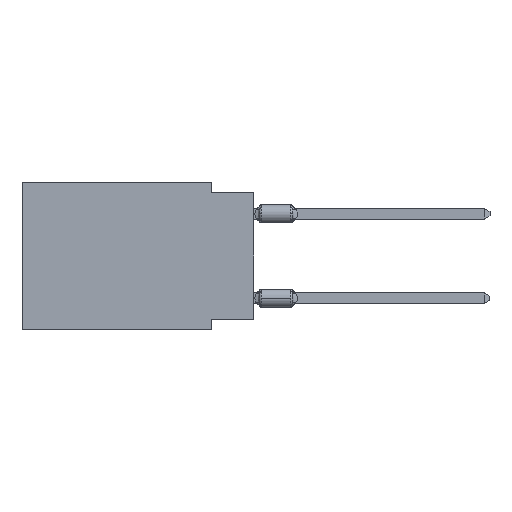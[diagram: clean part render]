
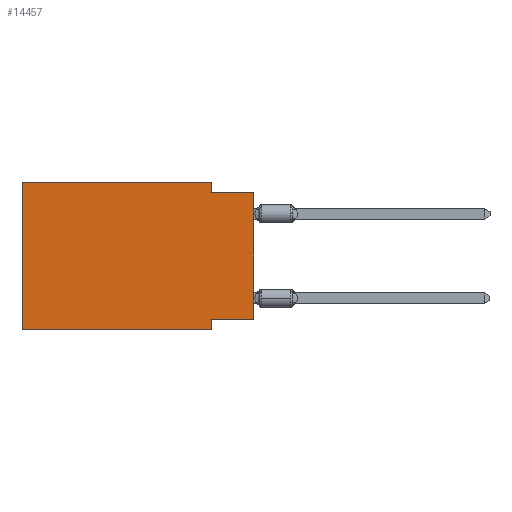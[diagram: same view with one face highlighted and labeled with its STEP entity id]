
A CAD part, left-side view. The second image highlights one B-rep face of the part: STEP entity #14457.
In plain terms, the highlighted planar face has unit normal (-1, 0, 0).
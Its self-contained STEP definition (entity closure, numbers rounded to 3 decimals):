
#102 = VERTEX_POINT ( 'NONE', #18695 ) ;
#424 = CARTESIAN_POINT ( 'NONE',  ( 0., 2.54, -0.635 ) ) ;
#1147 = ORIENTED_EDGE ( 'NONE', *, *, #19798, .F. ) ;
#1433 = LINE ( 'NONE', #1546, #9938 ) ;
#1546 = CARTESIAN_POINT ( 'NONE',  ( 0., 13.97, 0. ) ) ;
#1743 = CARTESIAN_POINT ( 'NONE',  ( 0., 2.54, 0. ) ) ;
#1990 = DIRECTION ( 'NONE',  ( 0., 0., 1. ) ) ;
#2003 = ORIENTED_EDGE ( 'NONE', *, *, #21666, .T. ) ;
#2311 = ORIENTED_EDGE ( 'NONE', *, *, #20406, .F. ) ;
#2910 = CARTESIAN_POINT ( 'NONE',  ( 0., 0., -8.255 ) ) ;
#2948 = DIRECTION ( 'NONE',  ( 0., -1., 0. ) ) ;
#3530 = ORIENTED_EDGE ( 'NONE', *, *, #18967, .F. ) ;
#4427 = CARTESIAN_POINT ( 'NONE',  ( 0., 13.97, -8.89 ) ) ;
#4794 = VERTEX_POINT ( 'NONE', #21587 ) ;
#4802 = VECTOR ( 'NONE', #16506, 1000. ) ;
#5285 = PLANE ( 'NONE',  #20352 ) ;
#5756 = LINE ( 'NONE', #11110, #18451 ) ;
#6217 = EDGE_CURVE ( 'NONE', #4794, #23227, #7727, .T. ) ;
#6686 = DIRECTION ( 'NONE',  ( 0., 0., -1. ) ) ;
#6759 = LINE ( 'NONE', #21975, #4802 ) ;
#6980 = VECTOR ( 'NONE', #1990, 1000. ) ;
#6994 = EDGE_LOOP ( 'NONE', ( #9531, #3530, #1147, #10972, #20057, #2003, #19799, #2311 ) ) ;
#7727 = LINE ( 'NONE', #15343, #6980 ) ;
#8943 = VERTEX_POINT ( 'NONE', #11607 ) ;
#8981 = DIRECTION ( 'NONE',  ( 0., 0., -1. ) ) ;
#9531 = ORIENTED_EDGE ( 'NONE', *, *, #6217, .T. ) ;
#9938 = VECTOR ( 'NONE', #14885, 1000. ) ;
#10057 = EDGE_CURVE ( 'NONE', #8943, #102, #16176, .T. ) ;
#10509 = DIRECTION ( 'NONE',  ( 0., 1., 0. ) ) ;
#10972 = ORIENTED_EDGE ( 'NONE', *, *, #24238, .F. ) ;
#11110 = CARTESIAN_POINT ( 'NONE',  ( 0., 13.97, 0. ) ) ;
#11607 = CARTESIAN_POINT ( 'NONE',  ( 0., 2.54, -8.255 ) ) ;
#12428 = CARTESIAN_POINT ( 'NONE',  ( 0., 13.97, 0. ) ) ;
#12641 = DIRECTION ( 'NONE',  ( 1., 0., 0. ) ) ;
#12744 = LINE ( 'NONE', #2910, #23574 ) ;
#12770 = VERTEX_POINT ( 'NONE', #18416 ) ;
#14263 = CARTESIAN_POINT ( 'NONE',  ( 0., 13.97, 0. ) ) ;
#14457 = ADVANCED_FACE ( 'NONE', ( #14522 ), #5285, .F. ) ;
#14522 = FACE_OUTER_BOUND ( 'NONE', #6994, .T. ) ;
#14885 = DIRECTION ( 'NONE',  ( 0., -1., 0. ) ) ;
#15343 = CARTESIAN_POINT ( 'NONE',  ( 0., 0., 0. ) ) ;
#16173 = CARTESIAN_POINT ( 'NONE',  ( 0., 2.54, 0. ) ) ;
#16176 = LINE ( 'NONE', #23762, #17818 ) ;
#16506 = DIRECTION ( 'NONE',  ( 0., -1., 0. ) ) ;
#17249 = VERTEX_POINT ( 'NONE', #424 ) ;
#17818 = VECTOR ( 'NONE', #6686, 1000. ) ;
#18416 = CARTESIAN_POINT ( 'NONE',  ( 0., 13.97, -8.89 ) ) ;
#18451 = VECTOR ( 'NONE', #18727, 1000. ) ;
#18695 = CARTESIAN_POINT ( 'NONE',  ( 0., 2.54, -8.89 ) ) ;
#18727 = DIRECTION ( 'NONE',  ( 0., 0., 1. ) ) ;
#18871 = VECTOR ( 'NONE', #2948, 1000. ) ;
#18967 = EDGE_CURVE ( 'NONE', #17249, #23227, #6759, .T. ) ;
#19798 = EDGE_CURVE ( 'NONE', #22884, #17249, #20569, .T. ) ;
#19799 = ORIENTED_EDGE ( 'NONE', *, *, #10057, .F. ) ;
#20057 = ORIENTED_EDGE ( 'NONE', *, *, #20559, .F. ) ;
#20257 = DIRECTION ( 'NONE',  ( 0., 0., -1. ) ) ;
#20352 = AXIS2_PLACEMENT_3D ( 'NONE', #14263, #12641, #20257 ) ;
#20406 = EDGE_CURVE ( 'NONE', #4794, #8943, #12744, .T. ) ;
#20559 = EDGE_CURVE ( 'NONE', #12770, #23717, #5756, .T. ) ;
#20569 = LINE ( 'NONE', #1743, #20769 ) ;
#20769 = VECTOR ( 'NONE', #8981, 1000. ) ;
#21559 = CARTESIAN_POINT ( 'NONE',  ( 0., 0., -0.635 ) ) ;
#21587 = CARTESIAN_POINT ( 'NONE',  ( 0., 0., -8.255 ) ) ;
#21666 = EDGE_CURVE ( 'NONE', #12770, #102, #21883, .T. ) ;
#21883 = LINE ( 'NONE', #4427, #18871 ) ;
#21975 = CARTESIAN_POINT ( 'NONE',  ( 0., 0., -0.635 ) ) ;
#22884 = VERTEX_POINT ( 'NONE', #16173 ) ;
#23227 = VERTEX_POINT ( 'NONE', #21559 ) ;
#23574 = VECTOR ( 'NONE', #10509, 1000. ) ;
#23717 = VERTEX_POINT ( 'NONE', #12428 ) ;
#23762 = CARTESIAN_POINT ( 'NONE',  ( 0., 2.54, -8.89 ) ) ;
#24238 = EDGE_CURVE ( 'NONE', #23717, #22884, #1433, .T. ) ;
